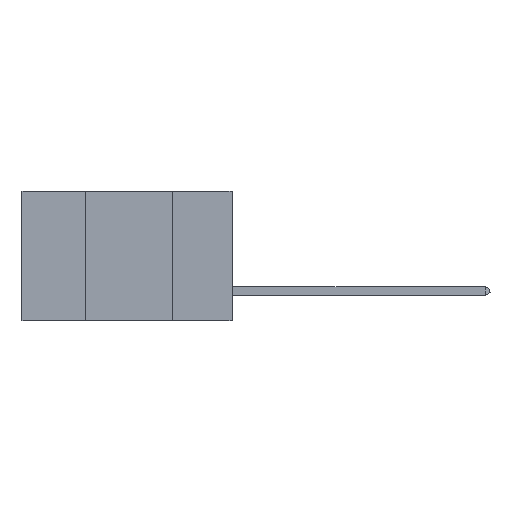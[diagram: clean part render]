
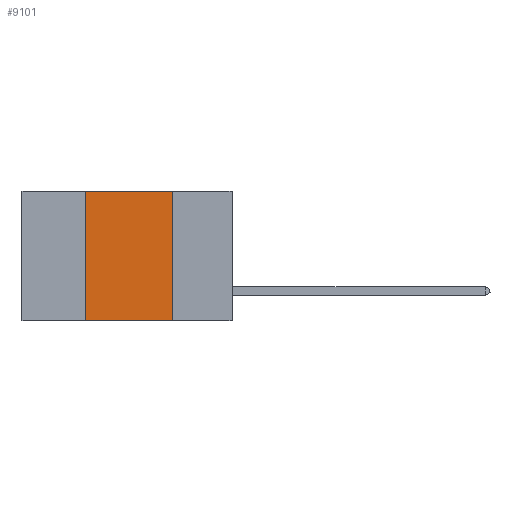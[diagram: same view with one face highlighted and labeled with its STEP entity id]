
A CAD part, left-side view. The second image highlights one B-rep face of the part: STEP entity #9101.
In plain terms, the highlighted planar face has unit normal (-1, 0, 0).
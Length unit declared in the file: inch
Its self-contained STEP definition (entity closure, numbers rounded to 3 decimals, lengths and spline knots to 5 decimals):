
#146 = VECTOR ( 'NONE', #522, 39.37008 ) ;
#522 = DIRECTION ( 'NONE',  ( 0., -1., 0. ) ) ;
#765 = VECTOR ( 'NONE', #9844, 39.37008 ) ;
#1452 = EDGE_CURVE ( 'NONE', #19080, #9598, #14955, .T. ) ;
#1833 = EDGE_LOOP ( 'NONE', ( #16001, #4431, #20635, #7676 ) ) ;
#1958 = VECTOR ( 'NONE', #11407, 39.37008 ) ;
#2156 = CARTESIAN_POINT ( 'NONE',  ( 0., 0.6, -0.37 ) ) ;
#2262 = VERTEX_POINT ( 'NONE', #2560 ) ;
#2346 = CARTESIAN_POINT ( 'NONE',  ( 0., 0.42, -0.37 ) ) ;
#2560 = CARTESIAN_POINT ( 'NONE',  ( 0., 0.17, 0. ) ) ;
#4431 = ORIENTED_EDGE ( 'NONE', *, *, #11613, .F. ) ;
#4475 = CARTESIAN_POINT ( 'NONE',  ( 0., 0.17, -0.37 ) ) ;
#5126 = EDGE_CURVE ( 'NONE', #19080, #11349, #11290, .T. ) ;
#6482 = CARTESIAN_POINT ( 'NONE',  ( 0., 0.17, 0. ) ) ;
#6742 = LINE ( 'NONE', #6482, #1958 ) ;
#7202 = DIRECTION ( 'NONE',  ( 0., -1., 0. ) ) ;
#7303 = PLANE ( 'NONE',  #11997 ) ;
#7676 = ORIENTED_EDGE ( 'NONE', *, *, #5126, .T. ) ;
#9012 = CARTESIAN_POINT ( 'NONE',  ( 0., 0.6, 0. ) ) ;
#9101 = ADVANCED_FACE ( 'NONE', ( #19083 ), #7303, .F. ) ;
#9280 = LINE ( 'NONE', #20145, #146 ) ;
#9598 = VERTEX_POINT ( 'NONE', #10531 ) ;
#9844 = DIRECTION ( 'NONE',  ( 0., 0., 1. ) ) ;
#10089 = EDGE_CURVE ( 'NONE', #2262, #11349, #6742, .T. ) ;
#10531 = CARTESIAN_POINT ( 'NONE',  ( 0., 0.42, 0. ) ) ;
#11290 = LINE ( 'NONE', #2156, #14874 ) ;
#11349 = VERTEX_POINT ( 'NONE', #4475 ) ;
#11407 = DIRECTION ( 'NONE',  ( 0., 0., -1. ) ) ;
#11613 = EDGE_CURVE ( 'NONE', #9598, #2262, #9280, .T. ) ;
#11997 = AXIS2_PLACEMENT_3D ( 'NONE', #9012, #16918, #20445 ) ;
#14874 = VECTOR ( 'NONE', #7202, 39.37008 ) ;
#14955 = LINE ( 'NONE', #17856, #765 ) ;
#16001 = ORIENTED_EDGE ( 'NONE', *, *, #10089, .F. ) ;
#16918 = DIRECTION ( 'NONE',  ( 1., 0., 0. ) ) ;
#17856 = CARTESIAN_POINT ( 'NONE',  ( 0., 0.42, 0. ) ) ;
#19080 = VERTEX_POINT ( 'NONE', #2346 ) ;
#19083 = FACE_OUTER_BOUND ( 'NONE', #1833, .T. ) ;
#20145 = CARTESIAN_POINT ( 'NONE',  ( 0., 0.6, 0. ) ) ;
#20445 = DIRECTION ( 'NONE',  ( 0., 0., -1. ) ) ;
#20635 = ORIENTED_EDGE ( 'NONE', *, *, #1452, .F. ) ;
